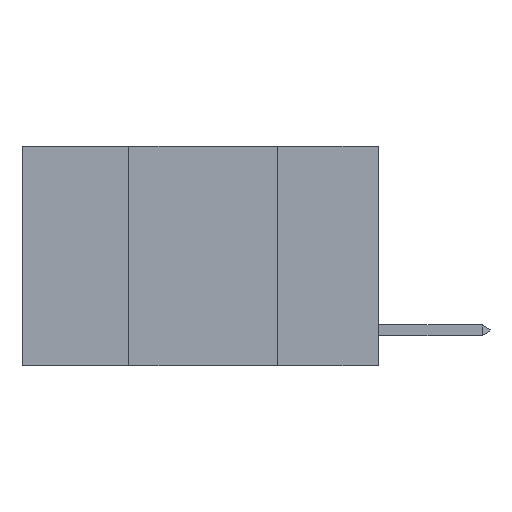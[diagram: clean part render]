
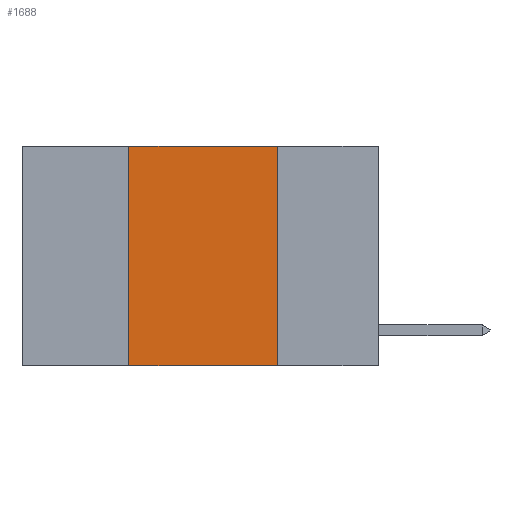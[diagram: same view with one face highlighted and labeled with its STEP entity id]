
A CAD part, left-side view. The second image highlights one B-rep face of the part: STEP entity #1688.
In plain terms, the highlighted planar face has unit normal (-1, 0, 0).
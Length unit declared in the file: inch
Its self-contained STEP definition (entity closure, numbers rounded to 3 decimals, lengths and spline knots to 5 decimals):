
#435 = VECTOR ( 'NONE', #9917, 39.37008 ) ;
#508 = ORIENTED_EDGE ( 'NONE', *, *, #6422, .T. ) ;
#531 = DIRECTION ( 'NONE',  ( 0., -1., 0. ) ) ;
#812 = PLANE ( 'NONE',  #2989 ) ;
#1622 = FACE_OUTER_BOUND ( 'NONE', #1886, .T. ) ;
#1688 = ADVANCED_FACE ( 'NONE', ( #1622 ), #812, .F. ) ;
#1722 = VERTEX_POINT ( 'NONE', #4269 ) ;
#1859 = CARTESIAN_POINT ( 'NONE',  ( 0., 0.17, 0. ) ) ;
#1886 = EDGE_LOOP ( 'NONE', ( #11472, #10315, #3669, #508 ) ) ;
#1942 = DIRECTION ( 'NONE',  ( 0., 0., -1. ) ) ;
#1972 = EDGE_CURVE ( 'NONE', #6657, #1722, #11247, .T. ) ;
#2989 = AXIS2_PLACEMENT_3D ( 'NONE', #4381, #7991, #11630 ) ;
#3189 = VECTOR ( 'NONE', #10438, 39.37008 ) ;
#3669 = ORIENTED_EDGE ( 'NONE', *, *, #1972, .F. ) ;
#4205 = LINE ( 'NONE', #7189, #435 ) ;
#4231 = CARTESIAN_POINT ( 'NONE',  ( 0., 0.6, -0.37 ) ) ;
#4269 = CARTESIAN_POINT ( 'NONE',  ( 0., 0.42, 0. ) ) ;
#4288 = LINE ( 'NONE', #4231, #5014 ) ;
#4381 = CARTESIAN_POINT ( 'NONE',  ( 0., 0.6, 0. ) ) ;
#4415 = EDGE_CURVE ( 'NONE', #1722, #8391, #4205, .T. ) ;
#4516 = CARTESIAN_POINT ( 'NONE',  ( 0., 0.17, 0. ) ) ;
#4517 = VECTOR ( 'NONE', #1942, 39.37008 ) ;
#5014 = VECTOR ( 'NONE', #531, 39.37008 ) ;
#5832 = CARTESIAN_POINT ( 'NONE',  ( 0., 0.17, -0.37 ) ) ;
#6422 = EDGE_CURVE ( 'NONE', #6657, #8169, #4288, .T. ) ;
#6657 = VERTEX_POINT ( 'NONE', #7037 ) ;
#7037 = CARTESIAN_POINT ( 'NONE',  ( 0., 0.42, -0.37 ) ) ;
#7189 = CARTESIAN_POINT ( 'NONE',  ( 0., 0.6, 0. ) ) ;
#7548 = CARTESIAN_POINT ( 'NONE',  ( 0., 0.42, 0. ) ) ;
#7991 = DIRECTION ( 'NONE',  ( 1., 0., 0. ) ) ;
#8169 = VERTEX_POINT ( 'NONE', #5832 ) ;
#8391 = VERTEX_POINT ( 'NONE', #1859 ) ;
#9917 = DIRECTION ( 'NONE',  ( 0., -1., 0. ) ) ;
#10125 = EDGE_CURVE ( 'NONE', #8391, #8169, #11599, .T. ) ;
#10315 = ORIENTED_EDGE ( 'NONE', *, *, #4415, .F. ) ;
#10438 = DIRECTION ( 'NONE',  ( 0., 0., 1. ) ) ;
#11247 = LINE ( 'NONE', #7548, #3189 ) ;
#11472 = ORIENTED_EDGE ( 'NONE', *, *, #10125, .F. ) ;
#11599 = LINE ( 'NONE', #4516, #4517 ) ;
#11630 = DIRECTION ( 'NONE',  ( 0., 0., -1. ) ) ;
